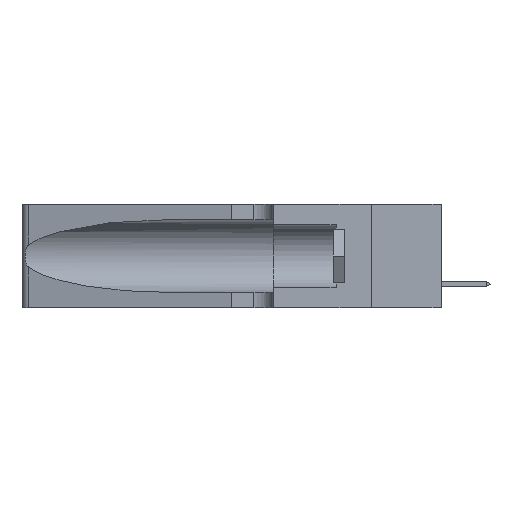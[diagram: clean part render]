
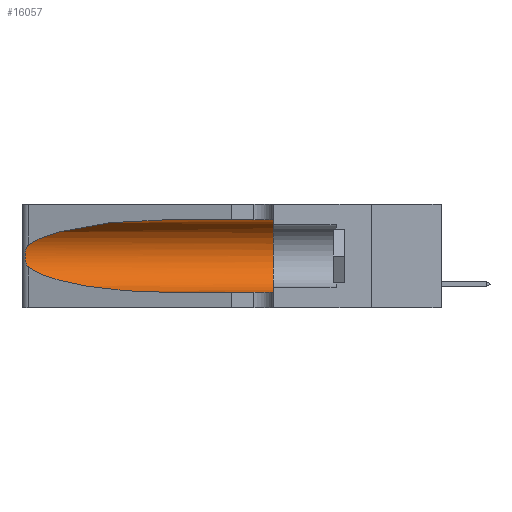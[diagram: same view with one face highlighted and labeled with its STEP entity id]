
A CAD part, left-side view. The second image highlights one B-rep face of the part: STEP entity #16057.
In plain terms, the highlighted cylindrical face has radius 3.308 mm (diameter 6.617 mm), a partial arc.
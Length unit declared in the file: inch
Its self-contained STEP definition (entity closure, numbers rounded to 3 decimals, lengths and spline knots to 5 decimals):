
#59 = ORIENTED_EDGE ( 'NONE', *, *, #7804, .T. ) ;
#225 = CARTESIAN_POINT ( 'NONE',  ( 0.1305, 0.35, 0.185 ) ) ;
#234 =( BOUNDED_CURVE ( )  B_SPLINE_CURVE ( 3, ( #8026, #6649, #11210, #8248 ),
 .UNSPECIFIED., .F., .T. ) 
 B_SPLINE_CURVE_WITH_KNOTS ( ( 4, 4 ),
 ( 1.5708, 2.84003 ),
 .UNSPECIFIED. ) 
 CURVE ( )  GEOMETRIC_REPRESENTATION_ITEM ( )  RATIONAL_B_SPLINE_CURVE ( ( 1., 0.87, 0.87, 1. ) ) 
 REPRESENTATION_ITEM ( '' )  );
#968 = CARTESIAN_POINT ( 'NONE',  ( 0.26075, 1.23896, 0.178 ) ) ;
#1079 = EDGE_CURVE ( 'NONE', #4640, #19086, #8512, .T. ) ;
#1741 = CARTESIAN_POINT ( 'NONE',  ( 0.25487, 1.22718, 0.14631 ) ) ;
#1788 = CIRCLE ( 'NONE', #2710, 0.13025 ) ;
#1995 = ORIENTED_EDGE ( 'NONE', *, *, #2928, .T. ) ;
#2265 = CARTESIAN_POINT ( 'NONE',  ( 0.25856, 1.23593, 0.16098 ) ) ;
#2710 = AXIS2_PLACEMENT_3D ( 'NONE', #225, #9665, #15945 ) ;
#2928 = EDGE_CURVE ( 'NONE', #10764, #18651, #15033, .T. ) ;
#3109 = CYLINDRICAL_SURFACE ( 'NONE', #17359, 0.13025 ) ;
#3522 = CARTESIAN_POINT ( 'NONE',  ( 0.25639, 1.23184, 0.21858 ) ) ;
#4069 = CARTESIAN_POINT ( 'NONE',  ( 0.26018, 1.23835, 0.19895 ) ) ;
#4313 = FACE_OUTER_BOUND ( 'NONE', #12873, .T. ) ;
#4599 = DIRECTION ( 'NONE',  ( 0., -1., 0. ) ) ;
#4640 = VERTEX_POINT ( 'NONE', #18812 ) ;
#4881 = DIRECTION ( 'NONE',  ( 0., -1., 0. ) ) ;
#5198 = VECTOR ( 'NONE', #16575, 39.37008 ) ;
#5290 = CARTESIAN_POINT ( 'NONE',  ( 0.25487, 1.22718, 0.14631 ) ) ;
#6339 = CARTESIAN_POINT ( 'NONE',  ( 0.2373, 1.15595, 0.08982 ) ) ;
#6532 = VERTEX_POINT ( 'NONE', #11005 ) ;
#6649 = CARTESIAN_POINT ( 'NONE',  ( 0.18966, 0.96281, 0.31525 ) ) ;
#7277 = CARTESIAN_POINT ( 'NONE',  ( 0.26017, 1.23833, 0.17102 ) ) ;
#7551 = ORIENTED_EDGE ( 'NONE', *, *, #1079, .T. ) ;
#7804 = EDGE_CURVE ( 'NONE', #18651, #4640, #17791, .T. ) ;
#8026 = CARTESIAN_POINT ( 'NONE',  ( 0.1305, 0.72297, 0.31525 ) ) ;
#8248 = CARTESIAN_POINT ( 'NONE',  ( 0.25487, 1.22718, 0.22369 ) ) ;
#8512 = LINE ( 'NONE', #12406, #10239 ) ;
#8550 = CARTESIAN_POINT ( 'NONE',  ( 0.1305, 0.35, 0.05475 ) ) ;
#8617 = CARTESIAN_POINT ( 'NONE',  ( 0.25639, 1.23186, 0.15144 ) ) ;
#9665 = DIRECTION ( 'NONE',  ( 0., 1., 0. ) ) ;
#9753 = CARTESIAN_POINT ( 'NONE',  ( 0.1305, 0.72297, 0.05475 ) ) ;
#10129 = CARTESIAN_POINT ( 'NONE',  ( 0.25487, 1.22718, 0.22369 ) ) ;
#10239 = VECTOR ( 'NONE', #4599, 39.37008 ) ;
#10494 = CARTESIAN_POINT ( 'NONE',  ( 0.25487, 1.22718, 0.22369 ) ) ;
#10528 = CARTESIAN_POINT ( 'NONE',  ( 0.1305, 1.61858, 0.31525 ) ) ;
#10764 = VERTEX_POINT ( 'NONE', #10494 ) ;
#11005 = CARTESIAN_POINT ( 'NONE',  ( 0.1305, 0.35, 0.31525 ) ) ;
#11210 = CARTESIAN_POINT ( 'NONE',  ( 0.2373, 1.15595, 0.28018 ) ) ;
#11234 = CARTESIAN_POINT ( 'NONE',  ( 0.18966, 0.96281, 0.05475 ) ) ;
#11633 = CARTESIAN_POINT ( 'NONE',  ( 0.25555, 1.22994, 0.2215 ) ) ;
#11772 = ORIENTED_EDGE ( 'NONE', *, *, #18304, .F. ) ;
#11810 = ORIENTED_EDGE ( 'NONE', *, *, #19830, .T. ) ;
#12406 = CARTESIAN_POINT ( 'NONE',  ( 0.1305, 1.61858, 0.05475 ) ) ;
#12650 = EDGE_CURVE ( 'NONE', #14134, #6532, #14968, .T. ) ;
#12873 = EDGE_LOOP ( 'NONE', ( #11810, #1995, #59, #7551, #11772, #15699 ) ) ;
#14134 = VERTEX_POINT ( 'NONE', #14872 ) ;
#14872 = CARTESIAN_POINT ( 'NONE',  ( 0.1305, 0.72297, 0.31525 ) ) ;
#14968 = LINE ( 'NONE', #10528, #5198 ) ;
#14985 = CARTESIAN_POINT ( 'NONE',  ( 0.26075, 1.23896, 0.19203 ) ) ;
#15033 = B_SPLINE_CURVE_WITH_KNOTS ( 'NONE', 3,
 ( #10129, #11633, #3522, #16306, #17863, #4069, #14985, #968, #7277, #2265, #17927, #8617, #20078, #5290 ),
 .UNSPECIFIED., .F., .F.,
 ( 4, 2, 2, 2, 2, 2, 4 ),
 ( 0., 0.00027, 0.00053, 0.00107, 0.0016, 0.00187, 0.00214 ),
 .UNSPECIFIED. ) ;
#15619 = CARTESIAN_POINT ( 'NONE',  ( 0.1305, 1.61858, 0.185 ) ) ;
#15699 = ORIENTED_EDGE ( 'NONE', *, *, #12650, .F. ) ;
#15945 = DIRECTION ( 'NONE',  ( 0., 0., 1. ) ) ;
#16057 = ADVANCED_FACE ( 'NONE', ( #4313 ), #3109, .F. ) ;
#16306 = CARTESIAN_POINT ( 'NONE',  ( 0.25787, 1.23484, 0.2124 ) ) ;
#16575 = DIRECTION ( 'NONE',  ( 0., -1., 0. ) ) ;
#17359 = AXIS2_PLACEMENT_3D ( 'NONE', #15619, #4881, #17508 ) ;
#17508 = DIRECTION ( 'NONE',  ( 0., 0., -1. ) ) ;
#17550 = CARTESIAN_POINT ( 'NONE',  ( 0.25487, 1.22718, 0.14631 ) ) ;
#17791 =( BOUNDED_CURVE ( )  B_SPLINE_CURVE ( 3, ( #1741, #6339, #11234, #9753 ),
 .UNSPECIFIED., .F., .F. ) 
 B_SPLINE_CURVE_WITH_KNOTS ( ( 4, 4 ),
 ( 3.44316, 4.71239 ),
 .UNSPECIFIED. ) 
 CURVE ( )  GEOMETRIC_REPRESENTATION_ITEM ( )  RATIONAL_B_SPLINE_CURVE ( ( 1., 0.87, 0.87, 1. ) ) 
 REPRESENTATION_ITEM ( '' )  );
#17863 = CARTESIAN_POINT ( 'NONE',  ( 0.25854, 1.2359, 0.20912 ) ) ;
#17927 = CARTESIAN_POINT ( 'NONE',  ( 0.25789, 1.23486, 0.15765 ) ) ;
#18304 = EDGE_CURVE ( 'NONE', #6532, #19086, #1788, .T. ) ;
#18651 = VERTEX_POINT ( 'NONE', #17550 ) ;
#18812 = CARTESIAN_POINT ( 'NONE',  ( 0.1305, 0.72297, 0.05475 ) ) ;
#19086 = VERTEX_POINT ( 'NONE', #8550 ) ;
#19830 = EDGE_CURVE ( 'NONE', #14134, #10764, #234, .T. ) ;
#20078 = CARTESIAN_POINT ( 'NONE',  ( 0.25555, 1.22993, 0.14849 ) ) ;
